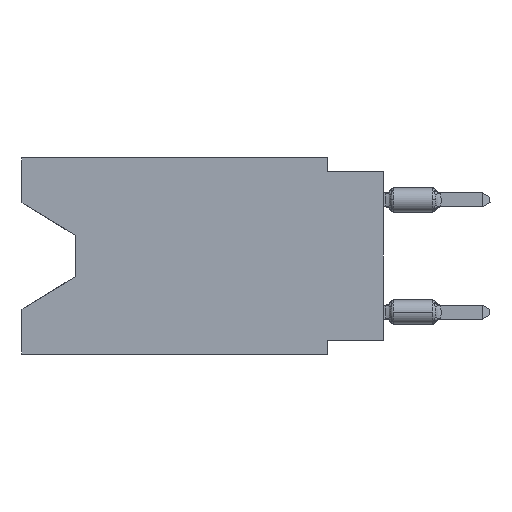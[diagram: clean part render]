
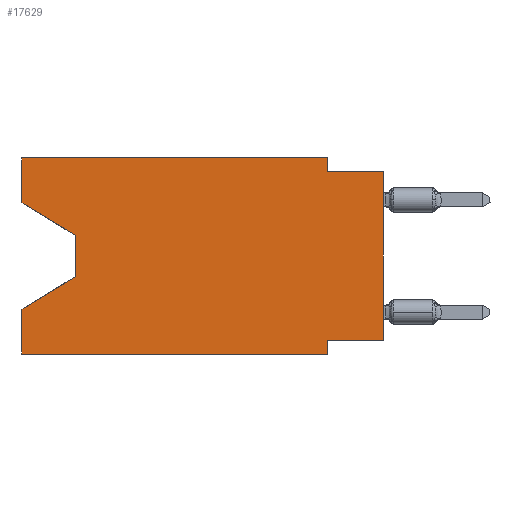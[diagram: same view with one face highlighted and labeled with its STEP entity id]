
A CAD part, left-side view. The second image highlights one B-rep face of the part: STEP entity #17629.
In plain terms, the highlighted planar face has unit normal (-1, 0, 0).
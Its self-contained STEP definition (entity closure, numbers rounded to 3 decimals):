
#694 = VERTEX_POINT ( 'NONE', #1748 ) ;
#922 = VERTEX_POINT ( 'NONE', #1080 ) ;
#1080 = CARTESIAN_POINT ( 'NONE',  ( 0., 13.97, -3.505 ) ) ;
#1322 = CARTESIAN_POINT ( 'NONE',  ( 0., 2.54, 0. ) ) ;
#1478 = EDGE_CURVE ( 'NONE', #11756, #2287, #5574, .T. ) ;
#1748 = CARTESIAN_POINT ( 'NONE',  ( 0., 16.383, -8.89 ) ) ;
#1775 = VERTEX_POINT ( 'NONE', #18099 ) ;
#2102 = VECTOR ( 'NONE', #19851, 1000. ) ;
#2287 = VERTEX_POINT ( 'NONE', #17390 ) ;
#2321 = DIRECTION ( 'NONE',  ( 0., 0., -1. ) ) ;
#2336 = ORIENTED_EDGE ( 'NONE', *, *, #18016, .F. ) ;
#2394 = CARTESIAN_POINT ( 'NONE',  ( 0., 16.383, 0. ) ) ;
#2947 = EDGE_LOOP ( 'NONE', ( #20136, #4622, #12012, #11713, #13268, #3580, #20964, #17098, #20162, #2336, #15123, #13793 ) ) ;
#3020 = VECTOR ( 'NONE', #14265, 1000. ) ;
#3096 = VECTOR ( 'NONE', #18609, 1000. ) ;
#3123 = DIRECTION ( 'NONE',  ( 0., 0.855, -0.519 ) ) ;
#3157 = VECTOR ( 'NONE', #20819, 1000. ) ;
#3523 = VECTOR ( 'NONE', #3123, 1000. ) ;
#3580 = ORIENTED_EDGE ( 'NONE', *, *, #14938, .F. ) ;
#4474 = VERTEX_POINT ( 'NONE', #18795 ) ;
#4622 = ORIENTED_EDGE ( 'NONE', *, *, #12599, .T. ) ;
#4625 = PLANE ( 'NONE',  #10050 ) ;
#4808 = CARTESIAN_POINT ( 'NONE',  ( 0., 16.383, -8.89 ) ) ;
#4922 = EDGE_CURVE ( 'NONE', #4474, #10349, #12220, .T. ) ;
#5574 = LINE ( 'NONE', #18554, #6786 ) ;
#5945 = FACE_OUTER_BOUND ( 'NONE', #2947, .T. ) ;
#6097 = LINE ( 'NONE', #14596, #19446 ) ;
#6417 = CARTESIAN_POINT ( 'NONE',  ( 0., 16.383, -2.038 ) ) ;
#6707 = LINE ( 'NONE', #13363, #3523 ) ;
#6786 = VECTOR ( 'NONE', #20079, 1000. ) ;
#8367 = CARTESIAN_POINT ( 'NONE',  ( 0., 2.54, -0.635 ) ) ;
#8889 = EDGE_CURVE ( 'NONE', #16866, #4474, #14477, .T. ) ;
#9062 = VERTEX_POINT ( 'NONE', #8367 ) ;
#9375 = DIRECTION ( 'NONE',  ( 0., 1., 0. ) ) ;
#9493 = CARTESIAN_POINT ( 'NONE',  ( 0., 2.54, -8.89 ) ) ;
#10002 = LINE ( 'NONE', #20239, #19620 ) ;
#10050 = AXIS2_PLACEMENT_3D ( 'NONE', #14221, #10870, #19129 ) ;
#10264 = EDGE_CURVE ( 'NONE', #9062, #2287, #19525, .T. ) ;
#10349 = VERTEX_POINT ( 'NONE', #1322 ) ;
#10614 = LINE ( 'NONE', #17251, #18396 ) ;
#10671 = VECTOR ( 'NONE', #12881, 1000. ) ;
#10862 = CARTESIAN_POINT ( 'NONE',  ( 0., 13.97, -3.505 ) ) ;
#10870 = DIRECTION ( 'NONE',  ( 1., 0., 0. ) ) ;
#10904 = CARTESIAN_POINT ( 'NONE',  ( 0., 16.383, 0. ) ) ;
#11262 = LINE ( 'NONE', #10862, #14292 ) ;
#11713 = ORIENTED_EDGE ( 'NONE', *, *, #19716, .F. ) ;
#11756 = VERTEX_POINT ( 'NONE', #21140 ) ;
#12012 = ORIENTED_EDGE ( 'NONE', *, *, #13618, .T. ) ;
#12220 = LINE ( 'NONE', #2394, #3157 ) ;
#12446 = VERTEX_POINT ( 'NONE', #20326 ) ;
#12599 = EDGE_CURVE ( 'NONE', #922, #16057, #11262, .T. ) ;
#12789 = EDGE_CURVE ( 'NONE', #694, #19155, #13204, .T. ) ;
#12881 = DIRECTION ( 'NONE',  ( 0., -1., 0. ) ) ;
#13204 = LINE ( 'NONE', #4808, #2102 ) ;
#13268 = ORIENTED_EDGE ( 'NONE', *, *, #12789, .T. ) ;
#13363 = CARTESIAN_POINT ( 'NONE',  ( 0., 13.97, -5.385 ) ) ;
#13595 = DIRECTION ( 'NONE',  ( 0., 0., 1. ) ) ;
#13618 = EDGE_CURVE ( 'NONE', #16057, #12446, #6707, .T. ) ;
#13661 = LINE ( 'NONE', #20303, #18422 ) ;
#13793 = ORIENTED_EDGE ( 'NONE', *, *, #8889, .F. ) ;
#14031 = CARTESIAN_POINT ( 'NONE',  ( 0., 16.383, -2.038 ) ) ;
#14221 = CARTESIAN_POINT ( 'NONE',  ( 0., 16.383, 0. ) ) ;
#14265 = DIRECTION ( 'NONE',  ( 0., 0., 1. ) ) ;
#14292 = VECTOR ( 'NONE', #20758, 1000. ) ;
#14396 = EDGE_CURVE ( 'NONE', #11756, #1775, #6097, .T. ) ;
#14477 = LINE ( 'NONE', #10904, #3020 ) ;
#14596 = CARTESIAN_POINT ( 'NONE',  ( 0., 0., -8.255 ) ) ;
#14659 = EDGE_CURVE ( 'NONE', #16866, #922, #20581, .T. ) ;
#14938 = EDGE_CURVE ( 'NONE', #1775, #19155, #13661, .T. ) ;
#15123 = ORIENTED_EDGE ( 'NONE', *, *, #4922, .F. ) ;
#15396 = DIRECTION ( 'NONE',  ( 0., 0., -1. ) ) ;
#16057 = VERTEX_POINT ( 'NONE', #17628 ) ;
#16866 = VERTEX_POINT ( 'NONE', #6417 ) ;
#17098 = ORIENTED_EDGE ( 'NONE', *, *, #1478, .T. ) ;
#17251 = CARTESIAN_POINT ( 'NONE',  ( 0., 2.54, 0. ) ) ;
#17390 = CARTESIAN_POINT ( 'NONE',  ( 0., 0., -0.635 ) ) ;
#17628 = CARTESIAN_POINT ( 'NONE',  ( 0., 13.97, -5.385 ) ) ;
#17629 = ADVANCED_FACE ( 'NONE', ( #5945 ), #4625, .F. ) ;
#18016 = EDGE_CURVE ( 'NONE', #10349, #9062, #10614, .T. ) ;
#18099 = CARTESIAN_POINT ( 'NONE',  ( 0., 2.54, -8.255 ) ) ;
#18396 = VECTOR ( 'NONE', #2321, 1000. ) ;
#18422 = VECTOR ( 'NONE', #15396, 1000. ) ;
#18554 = CARTESIAN_POINT ( 'NONE',  ( 0., 0., 0. ) ) ;
#18609 = DIRECTION ( 'NONE',  ( 0., -0.855, -0.519 ) ) ;
#18795 = CARTESIAN_POINT ( 'NONE',  ( 0., 16.383, 0. ) ) ;
#19129 = DIRECTION ( 'NONE',  ( 0., 0., -1. ) ) ;
#19155 = VERTEX_POINT ( 'NONE', #9493 ) ;
#19446 = VECTOR ( 'NONE', #9375, 1000. ) ;
#19525 = LINE ( 'NONE', #21049, #10671 ) ;
#19620 = VECTOR ( 'NONE', #13595, 1000. ) ;
#19716 = EDGE_CURVE ( 'NONE', #694, #12446, #10002, .T. ) ;
#19851 = DIRECTION ( 'NONE',  ( 0., -1., 0. ) ) ;
#20079 = DIRECTION ( 'NONE',  ( 0., 0., 1. ) ) ;
#20136 = ORIENTED_EDGE ( 'NONE', *, *, #14659, .T. ) ;
#20162 = ORIENTED_EDGE ( 'NONE', *, *, #10264, .F. ) ;
#20239 = CARTESIAN_POINT ( 'NONE',  ( 0., 16.383, 0. ) ) ;
#20303 = CARTESIAN_POINT ( 'NONE',  ( 0., 2.54, -8.89 ) ) ;
#20326 = CARTESIAN_POINT ( 'NONE',  ( 0., 16.383, -6.852 ) ) ;
#20581 = LINE ( 'NONE', #14031, #3096 ) ;
#20758 = DIRECTION ( 'NONE',  ( 0., 0., -1. ) ) ;
#20819 = DIRECTION ( 'NONE',  ( 0., -1., 0. ) ) ;
#20964 = ORIENTED_EDGE ( 'NONE', *, *, #14396, .F. ) ;
#21049 = CARTESIAN_POINT ( 'NONE',  ( 0., 0., -0.635 ) ) ;
#21140 = CARTESIAN_POINT ( 'NONE',  ( 0., 0., -8.255 ) ) ;
